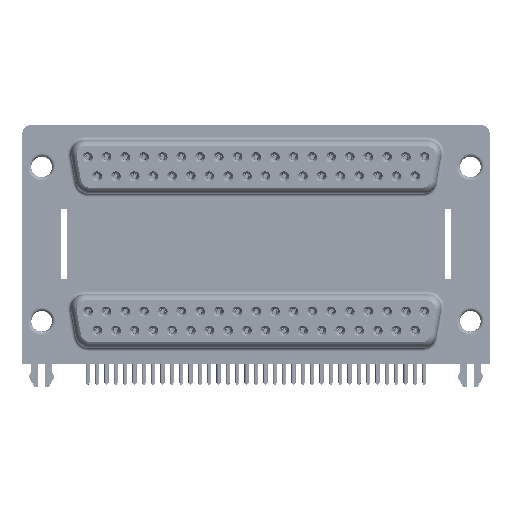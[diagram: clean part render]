
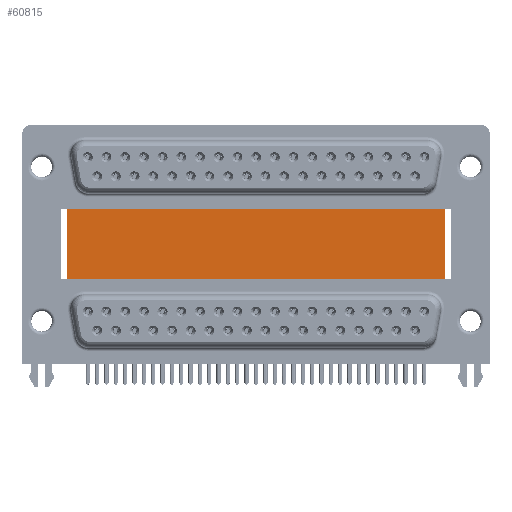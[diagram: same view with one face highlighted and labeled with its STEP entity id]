
A CAD part, top view. The second image highlights one B-rep face of the part: STEP entity #60815.
In plain terms, the highlighted planar face has unit normal (0, 0, 1).
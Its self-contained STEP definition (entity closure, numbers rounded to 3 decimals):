
#3010 = VERTEX_POINT ( 'NONE', #7764 ) ;
#3663 = LINE ( 'NONE', #4384, #8905 ) ;
#4384 = CARTESIAN_POINT ( 'NONE',  ( 3.79, 16.585, -12. ) ) ;
#5974 = CARTESIAN_POINT ( 'NONE',  ( 59.71, 16.585, -12. ) ) ;
#7764 = CARTESIAN_POINT ( 'NONE',  ( 3.79, 16.585, -12. ) ) ;
#8905 = VECTOR ( 'NONE', #43278, 1000. ) ;
#10369 = VECTOR ( 'NONE', #31904, 1000. ) ;
#11740 = CARTESIAN_POINT ( 'NONE',  ( 3.79, -3.735, -12. ) ) ;
#12080 = VECTOR ( 'NONE', #53981, 1000. ) ;
#12431 = VERTEX_POINT ( 'NONE', #31504 ) ;
#14514 = DIRECTION ( 'NONE',  ( -1., 0., 0. ) ) ;
#14726 = LINE ( 'NONE', #37504, #10369 ) ;
#15359 = EDGE_CURVE ( 'NONE', #3010, #60425, #3663, .T. ) ;
#15470 = ORIENTED_EDGE ( 'NONE', *, *, #15359, .T. ) ;
#15602 = ORIENTED_EDGE ( 'NONE', *, *, #23305, .T. ) ;
#19017 = DIRECTION ( 'NONE',  ( 0., 0., -1. ) ) ;
#23305 = EDGE_CURVE ( 'NONE', #60425, #46884, #14726, .T. ) ;
#25273 = CARTESIAN_POINT ( 'NONE',  ( 59.71, -3.735, -12. ) ) ;
#25577 = LINE ( 'NONE', #37898, #12080 ) ;
#26654 = VECTOR ( 'NONE', #28813, 1000. ) ;
#28813 = DIRECTION ( 'NONE',  ( 0., -1., 0. ) ) ;
#28884 = ORIENTED_EDGE ( 'NONE', *, *, #68506, .F. ) ;
#29722 = EDGE_LOOP ( 'NONE', ( #15602, #28884, #69843, #15470 ) ) ;
#31504 = CARTESIAN_POINT ( 'NONE',  ( 59.71, 16.585, -12. ) ) ;
#31904 = DIRECTION ( 'NONE',  ( 1., 0., 0. ) ) ;
#37504 = CARTESIAN_POINT ( 'NONE',  ( 3.79, -3.735, -12. ) ) ;
#37898 = CARTESIAN_POINT ( 'NONE',  ( 3.79, 16.585, -12. ) ) ;
#43278 = DIRECTION ( 'NONE',  ( 0., -1., 0. ) ) ;
#46884 = VERTEX_POINT ( 'NONE', #25273 ) ;
#47381 = PLANE ( 'NONE',  #61888 ) ;
#53981 = DIRECTION ( 'NONE',  ( 1., 0., 0. ) ) ;
#54462 = FACE_OUTER_BOUND ( 'NONE', #29722, .T. ) ;
#55164 = EDGE_CURVE ( 'NONE', #3010, #12431, #25577, .T. ) ;
#57209 = LINE ( 'NONE', #5974, #26654 ) ;
#60425 = VERTEX_POINT ( 'NONE', #11740 ) ;
#60815 = ADVANCED_FACE ( 'NONE', ( #54462 ), #47381, .F. ) ;
#61888 = AXIS2_PLACEMENT_3D ( 'NONE', #64946, #19017, #14514 ) ;
#64946 = CARTESIAN_POINT ( 'NONE',  ( 3.79, 16.585, -12. ) ) ;
#68506 = EDGE_CURVE ( 'NONE', #12431, #46884, #57209, .T. ) ;
#69843 = ORIENTED_EDGE ( 'NONE', *, *, #55164, .F. ) ;
